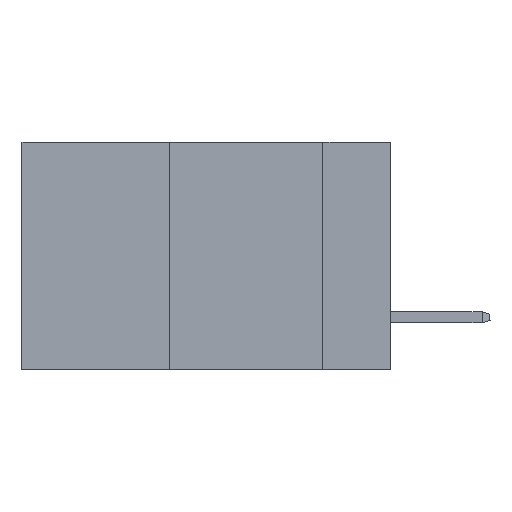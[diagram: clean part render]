
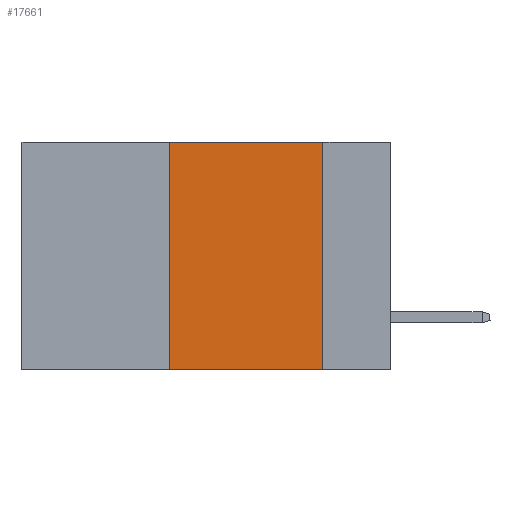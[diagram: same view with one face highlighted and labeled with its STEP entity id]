
A CAD part, left-side view. The second image highlights one B-rep face of the part: STEP entity #17661.
In plain terms, the highlighted planar face has unit normal (-1, 0, 0).
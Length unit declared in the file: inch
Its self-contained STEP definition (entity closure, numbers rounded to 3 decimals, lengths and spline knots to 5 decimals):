
#232 = VERTEX_POINT ( 'NONE', #8472 ) ;
#1068 = EDGE_CURVE ( 'NONE', #12991, #17829, #12032, .T. ) ;
#1323 = VECTOR ( 'NONE', #12175, 39.37008 ) ;
#2014 = CARTESIAN_POINT ( 'NONE',  ( 0., 0.11, -0.37 ) ) ;
#2426 = ORIENTED_EDGE ( 'NONE', *, *, #10227, .F. ) ;
#2608 = DIRECTION ( 'NONE',  ( 0., 0., -1. ) ) ;
#2906 = ORIENTED_EDGE ( 'NONE', *, *, #1068, .F. ) ;
#4775 = VERTEX_POINT ( 'NONE', #15894 ) ;
#4838 = CARTESIAN_POINT ( 'NONE',  ( 0., 0.6, -0.37 ) ) ;
#5638 = ORIENTED_EDGE ( 'NONE', *, *, #20474, .T. ) ;
#5878 = LINE ( 'NONE', #21677, #10193 ) ;
#6291 = DIRECTION ( 'NONE',  ( 1., 0., 0. ) ) ;
#7508 = EDGE_LOOP ( 'NONE', ( #2906, #2426, #12479, #5638 ) ) ;
#7916 = LINE ( 'NONE', #4838, #1323 ) ;
#8272 = DIRECTION ( 'NONE',  ( 0., -1., 0. ) ) ;
#8472 = CARTESIAN_POINT ( 'NONE',  ( 0., 0.36, 0. ) ) ;
#10193 = VECTOR ( 'NONE', #8272, 39.37008 ) ;
#10227 = EDGE_CURVE ( 'NONE', #232, #12991, #5878, .T. ) ;
#11377 = EDGE_CURVE ( 'NONE', #4775, #232, #22706, .T. ) ;
#11762 = DIRECTION ( 'NONE',  ( 0., 0., 1. ) ) ;
#12032 = LINE ( 'NONE', #16850, #22905 ) ;
#12175 = DIRECTION ( 'NONE',  ( 0., -1., 0. ) ) ;
#12479 = ORIENTED_EDGE ( 'NONE', *, *, #11377, .F. ) ;
#12991 = VERTEX_POINT ( 'NONE', #21110 ) ;
#13827 = CARTESIAN_POINT ( 'NONE',  ( 0., 0.36, 0. ) ) ;
#14413 = VECTOR ( 'NONE', #11762, 39.37008 ) ;
#15424 = CARTESIAN_POINT ( 'NONE',  ( 0., 0.6, 0. ) ) ;
#15894 = CARTESIAN_POINT ( 'NONE',  ( 0., 0.36, -0.37 ) ) ;
#16850 = CARTESIAN_POINT ( 'NONE',  ( 0., 0.11, 0. ) ) ;
#16879 = PLANE ( 'NONE',  #23608 ) ;
#17661 = ADVANCED_FACE ( 'NONE', ( #23270 ), #16879, .F. ) ;
#17829 = VERTEX_POINT ( 'NONE', #2014 ) ;
#20474 = EDGE_CURVE ( 'NONE', #4775, #17829, #7916, .T. ) ;
#20770 = DIRECTION ( 'NONE',  ( 0., 0., -1. ) ) ;
#21110 = CARTESIAN_POINT ( 'NONE',  ( 0., 0.11, 0. ) ) ;
#21677 = CARTESIAN_POINT ( 'NONE',  ( 0., 0.6, 0. ) ) ;
#22706 = LINE ( 'NONE', #13827, #14413 ) ;
#22905 = VECTOR ( 'NONE', #20770, 39.37008 ) ;
#23270 = FACE_OUTER_BOUND ( 'NONE', #7508, .T. ) ;
#23608 = AXIS2_PLACEMENT_3D ( 'NONE', #15424, #6291, #2608 ) ;
